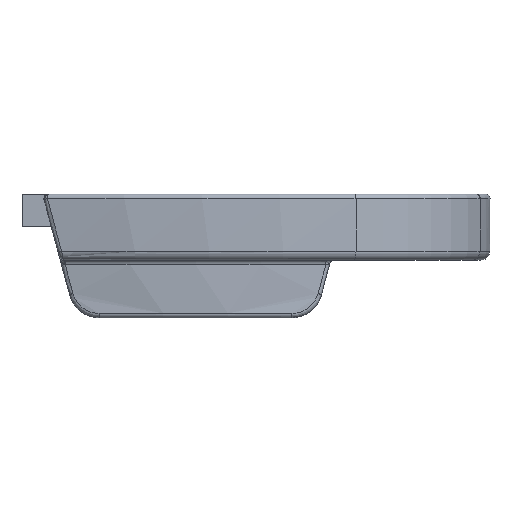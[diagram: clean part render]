
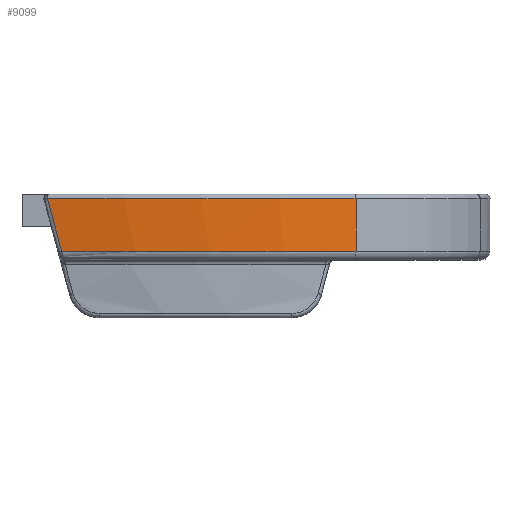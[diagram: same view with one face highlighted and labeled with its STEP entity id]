
A CAD part, front view. The second image highlights one B-rep face of the part: STEP entity #9099.
In plain terms, the highlighted cylindrical face has radius 57.404 mm (diameter 114.808 mm), a partial arc.
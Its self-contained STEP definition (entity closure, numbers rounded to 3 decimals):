
#77 = CIRCLE ( 'NONE', #2790, 57.404 ) ;
#321 = VERTEX_POINT ( 'NONE', #609 ) ;
#609 = CARTESIAN_POINT ( 'NONE',  ( 13.36, -14.405, -2.14 ) ) ;
#1017 = DIRECTION ( 'NONE',  ( -0.234, -0.972, 0. ) ) ;
#1640 = CARTESIAN_POINT ( 'NONE',  ( -13.612, -14.854, 0.982 ) ) ;
#1948 = CARTESIAN_POINT ( 'NONE',  ( -12.77, -15.035, -2.14 ) ) ;
#2167 = VERTEX_POINT ( 'NONE', #1948 ) ;
#2290 = CIRCLE ( 'NONE', #8801, 57.404 ) ;
#2571 = CARTESIAN_POINT ( 'NONE',  ( 13.36, -14.405, 2.537 ) ) ;
#2790 = AXIS2_PLACEMENT_3D ( 'NONE', #3219, #9717, #4161 ) ;
#2969 = ORIENTED_EDGE ( 'NONE', *, *, #9672, .T. ) ;
#3219 = CARTESIAN_POINT ( 'NONE',  ( -1.052, 41.161, 2.537 ) ) ;
#3844 = CARTESIAN_POINT ( 'NONE',  ( -1.052, 41.161, -2.14 ) ) ;
#3929 = EDGE_CURVE ( 'NONE', #321, #2167, #2290, .T. ) ;
#3995 = ORIENTED_EDGE ( 'NONE', *, *, #7634, .F. ) ;
#4161 = DIRECTION ( 'NONE',  ( 0.009, -1., 0. ) ) ;
#4728 = DIRECTION ( 'NONE',  ( 0., 0., 1. ) ) ;
#4795 = DIRECTION ( 'NONE',  ( 0.023, -1., 0. ) ) ;
#5267 = CYLINDRICAL_SURFACE ( 'NONE', #9690, 57.404 ) ;
#5355 = CARTESIAN_POINT ( 'NONE',  ( -13.191, -14.947, -0.577 ) ) ;
#5749 = VERTEX_POINT ( 'NONE', #6487 ) ;
#5834 = VECTOR ( 'NONE', #10350, 1000. ) ;
#6487 = CARTESIAN_POINT ( 'NONE',  ( -14.031, -14.757, 2.537 ) ) ;
#7180 = EDGE_CURVE ( 'NONE', #5749, #8158, #77, .T. ) ;
#7310 = ORIENTED_EDGE ( 'NONE', *, *, #7180, .F. ) ;
#7634 = EDGE_CURVE ( 'NONE', #2167, #5749, #12079, .T. ) ;
#8145 = CARTESIAN_POINT ( 'NONE',  ( -14.031, -14.757, 2.537 ) ) ;
#8147 = ORIENTED_EDGE ( 'NONE', *, *, #3929, .F. ) ;
#8158 = VERTEX_POINT ( 'NONE', #2571 ) ;
#8309 = LINE ( 'NONE', #9411, #5834 ) ;
#8801 = AXIS2_PLACEMENT_3D ( 'NONE', #3844, #10342, #4795 ) ;
#9099 = ADVANCED_FACE ( 'NONE', ( #10213 ), #5267, .T. ) ;
#9391 = EDGE_LOOP ( 'NONE', ( #3995, #8147, #2969, #7310 ) ) ;
#9411 = CARTESIAN_POINT ( 'NONE',  ( 13.36, -14.405, 0. ) ) ;
#9672 = EDGE_CURVE ( 'NONE', #321, #8158, #8309, .T. ) ;
#9690 = AXIS2_PLACEMENT_3D ( 'NONE', #11226, #4728, #1017 ) ;
#9717 = DIRECTION ( 'NONE',  ( 0., 0., 1. ) ) ;
#10213 = FACE_OUTER_BOUND ( 'NONE', #9391, .T. ) ;
#10342 = DIRECTION ( 'NONE',  ( 0., 0., -1. ) ) ;
#10350 = DIRECTION ( 'NONE',  ( 0., 0., 1. ) ) ;
#11226 = CARTESIAN_POINT ( 'NONE',  ( -1.052, 41.161, 0. ) ) ;
#11842 = CARTESIAN_POINT ( 'NONE',  ( -12.77, -15.035, -2.14 ) ) ;
#12079 =( BOUNDED_CURVE ( )  B_SPLINE_CURVE ( 3, ( #11842, #5355, #1640, #8145 ),
 .UNSPECIFIED., .F., .F. ) 
 B_SPLINE_CURVE_WITH_KNOTS ( ( 4, 4 ),
 ( 4.918, 4.94 ),
 .UNSPECIFIED. ) 
 CURVE ( )  GEOMETRIC_REPRESENTATION_ITEM ( )  RATIONAL_B_SPLINE_CURVE ( ( 1., 1., 1., 1. ) ) 
 REPRESENTATION_ITEM ( '' )  );
